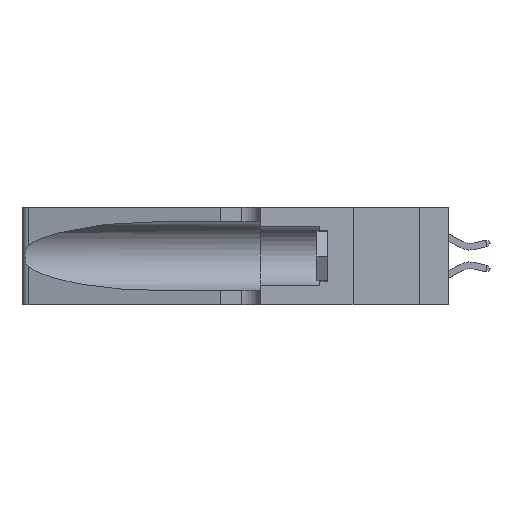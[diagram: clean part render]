
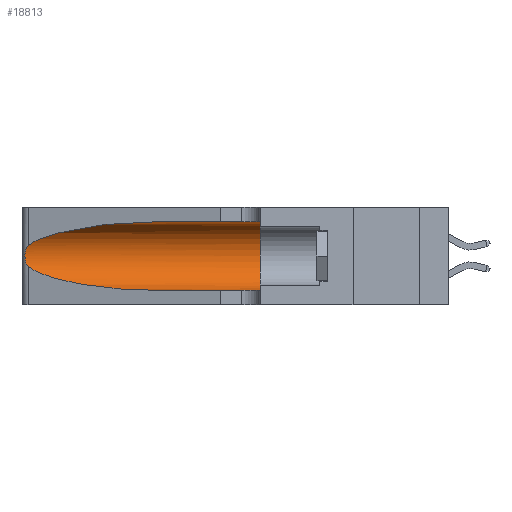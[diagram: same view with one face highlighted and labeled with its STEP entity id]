
A CAD part, left-side view. The second image highlights one B-rep face of the part: STEP entity #18813.
In plain terms, the highlighted cylindrical face has radius 3.308 mm (diameter 6.617 mm), a partial arc.
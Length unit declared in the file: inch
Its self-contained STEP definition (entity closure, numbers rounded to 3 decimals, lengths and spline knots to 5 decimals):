
#1074 = CARTESIAN_POINT ( 'NONE',  ( 0.1305, 0.35, 0.185 ) ) ;
#1989 = DIRECTION ( 'NONE',  ( 0., -1., 0. ) ) ;
#2255 = CARTESIAN_POINT ( 'NONE',  ( 0.26018, 1.23835, 0.19895 ) ) ;
#3294 = ORIENTED_EDGE ( 'NONE', *, *, #9250, .T. ) ;
#3367 = ORIENTED_EDGE ( 'NONE', *, *, #25952, .T. ) ;
#3958 = DIRECTION ( 'NONE',  ( 0., 0., 1. ) ) ;
#4105 = VERTEX_POINT ( 'NONE', #31030 ) ;
#4121 = EDGE_CURVE ( 'NONE', #25218, #33427, #22403, .T. ) ;
#5074 = CARTESIAN_POINT ( 'NONE',  ( 0.26075, 1.23896, 0.178 ) ) ;
#5595 = B_SPLINE_CURVE_WITH_KNOTS ( 'NONE', 3,
 ( #24106, #26830, #16064, #34982, #18802, #2255, #21521, #5074, #24222, #7913, #26949, #10658, #29675, #13404 ),
 .UNSPECIFIED., .F., .F.,
 ( 4, 2, 2, 2, 2, 2, 4 ),
 ( 0., 0.00027, 0.00053, 0.00107, 0.0016, 0.00187, 0.00214 ),
 .UNSPECIFIED. ) ;
#5622 = CARTESIAN_POINT ( 'NONE',  ( 0.25487, 1.22718, 0.14631 ) ) ;
#5791 = ORIENTED_EDGE ( 'NONE', *, *, #21318, .T. ) ;
#5900 = CARTESIAN_POINT ( 'NONE',  ( 0.1305, 0.72297, 0.31525 ) ) ;
#7913 = CARTESIAN_POINT ( 'NONE',  ( 0.25856, 1.23593, 0.16098 ) ) ;
#8551 = EDGE_CURVE ( 'NONE', #13097, #25218, #34399, .T. ) ;
#8970 = CARTESIAN_POINT ( 'NONE',  ( 0.1305, 0.35, 0.31525 ) ) ;
#9250 = EDGE_CURVE ( 'NONE', #13097, #4105, #11985, .T. ) ;
#9290 = CYLINDRICAL_SURFACE ( 'NONE', #19229, 0.13025 ) ;
#9618 = EDGE_CURVE ( 'NONE', #4105, #15932, #5595, .T. ) ;
#10658 = CARTESIAN_POINT ( 'NONE',  ( 0.25639, 1.23186, 0.15144 ) ) ;
#11782 = ORIENTED_EDGE ( 'NONE', *, *, #8551, .F. ) ;
#11954 = CARTESIAN_POINT ( 'NONE',  ( 0.1305, 0.72297, 0.05475 ) ) ;
#11985 =( BOUNDED_CURVE ( )  B_SPLINE_CURVE ( 3, ( #30616, #22592, #30732, #14511 ),
 .UNSPECIFIED., .F., .F. ) 
 B_SPLINE_CURVE_WITH_KNOTS ( ( 4, 4 ),
 ( 1.5708, 2.84003 ),
 .UNSPECIFIED. ) 
 CURVE ( )  GEOMETRIC_REPRESENTATION_ITEM ( )  RATIONAL_B_SPLINE_CURVE ( ( 1., 0.87, 0.87, 1. ) ) 
 REPRESENTATION_ITEM ( '' )  );
#12593 = VERTEX_POINT ( 'NONE', #11954 ) ;
#13097 = VERTEX_POINT ( 'NONE', #5900 ) ;
#13317 = ORIENTED_EDGE ( 'NONE', *, *, #9618, .T. ) ;
#13404 = CARTESIAN_POINT ( 'NONE',  ( 0.25487, 1.22718, 0.14631 ) ) ;
#13746 = CARTESIAN_POINT ( 'NONE',  ( 0.1305, 1.61858, 0.05475 ) ) ;
#14511 = CARTESIAN_POINT ( 'NONE',  ( 0.25487, 1.22718, 0.22369 ) ) ;
#14542 = CARTESIAN_POINT ( 'NONE',  ( 0.18966, 0.96281, 0.05475 ) ) ;
#15814 = CARTESIAN_POINT ( 'NONE',  ( 0.1305, 1.61858, 0.185 ) ) ;
#15932 = VERTEX_POINT ( 'NONE', #5622 ) ;
#16064 = CARTESIAN_POINT ( 'NONE',  ( 0.25639, 1.23184, 0.21858 ) ) ;
#16092 = EDGE_LOOP ( 'NONE', ( #3294, #13317, #3367, #5791, #34378, #11782 ) ) ;
#17302 = VECTOR ( 'NONE', #32702, 39.37008 ) ;
#18565 = DIRECTION ( 'NONE',  ( 0., 0., -1. ) ) ;
#18581 = CARTESIAN_POINT ( 'NONE',  ( 0.1305, 0.35, 0.05475 ) ) ;
#18802 = CARTESIAN_POINT ( 'NONE',  ( 0.25854, 1.2359, 0.20912 ) ) ;
#18813 = ADVANCED_FACE ( 'NONE', ( #23774 ), #9290, .F. ) ;
#19229 = AXIS2_PLACEMENT_3D ( 'NONE', #15814, #1989, #18565 ) ;
#19462 = CARTESIAN_POINT ( 'NONE',  ( 0.1305, 1.61858, 0.31525 ) ) ;
#20416 = DIRECTION ( 'NONE',  ( 0., 1., 0. ) ) ;
#21318 = EDGE_CURVE ( 'NONE', #12593, #33427, #31662, .T. ) ;
#21521 = CARTESIAN_POINT ( 'NONE',  ( 0.26075, 1.23896, 0.19203 ) ) ;
#22403 = CIRCLE ( 'NONE', #34010, 0.13025 ) ;
#22592 = CARTESIAN_POINT ( 'NONE',  ( 0.18966, 0.96281, 0.31525 ) ) ;
#22629 = CARTESIAN_POINT ( 'NONE',  ( 0.25487, 1.22718, 0.14631 ) ) ;
#23774 = FACE_OUTER_BOUND ( 'NONE', #16092, .T. ) ;
#24106 = CARTESIAN_POINT ( 'NONE',  ( 0.25487, 1.22718, 0.22369 ) ) ;
#24222 = CARTESIAN_POINT ( 'NONE',  ( 0.26017, 1.23833, 0.17102 ) ) ;
#25218 = VERTEX_POINT ( 'NONE', #8970 ) ;
#25733 =( BOUNDED_CURVE ( )  B_SPLINE_CURVE ( 3, ( #22629, #28067, #14542, #33492 ),
 .UNSPECIFIED., .F., .F. ) 
 B_SPLINE_CURVE_WITH_KNOTS ( ( 4, 4 ),
 ( 3.44316, 4.71239 ),
 .UNSPECIFIED. ) 
 CURVE ( )  GEOMETRIC_REPRESENTATION_ITEM ( )  RATIONAL_B_SPLINE_CURVE ( ( 1., 0.87, 0.87, 1. ) ) 
 REPRESENTATION_ITEM ( '' )  );
#25952 = EDGE_CURVE ( 'NONE', #15932, #12593, #25733, .T. ) ;
#26830 = CARTESIAN_POINT ( 'NONE',  ( 0.25555, 1.22994, 0.2215 ) ) ;
#26949 = CARTESIAN_POINT ( 'NONE',  ( 0.25789, 1.23486, 0.15765 ) ) ;
#27218 = VECTOR ( 'NONE', #30187, 39.37008 ) ;
#28067 = CARTESIAN_POINT ( 'NONE',  ( 0.2373, 1.15595, 0.08982 ) ) ;
#29675 = CARTESIAN_POINT ( 'NONE',  ( 0.25555, 1.22993, 0.14849 ) ) ;
#30187 = DIRECTION ( 'NONE',  ( 0., -1., 0. ) ) ;
#30616 = CARTESIAN_POINT ( 'NONE',  ( 0.1305, 0.72297, 0.31525 ) ) ;
#30732 = CARTESIAN_POINT ( 'NONE',  ( 0.2373, 1.15595, 0.28018 ) ) ;
#31030 = CARTESIAN_POINT ( 'NONE',  ( 0.25487, 1.22718, 0.22369 ) ) ;
#31662 = LINE ( 'NONE', #13746, #17302 ) ;
#32702 = DIRECTION ( 'NONE',  ( 0., -1., 0. ) ) ;
#33427 = VERTEX_POINT ( 'NONE', #18581 ) ;
#33492 = CARTESIAN_POINT ( 'NONE',  ( 0.1305, 0.72297, 0.05475 ) ) ;
#34010 = AXIS2_PLACEMENT_3D ( 'NONE', #1074, #20416, #3958 ) ;
#34378 = ORIENTED_EDGE ( 'NONE', *, *, #4121, .F. ) ;
#34399 = LINE ( 'NONE', #19462, #27218 ) ;
#34982 = CARTESIAN_POINT ( 'NONE',  ( 0.25787, 1.23484, 0.2124 ) ) ;
